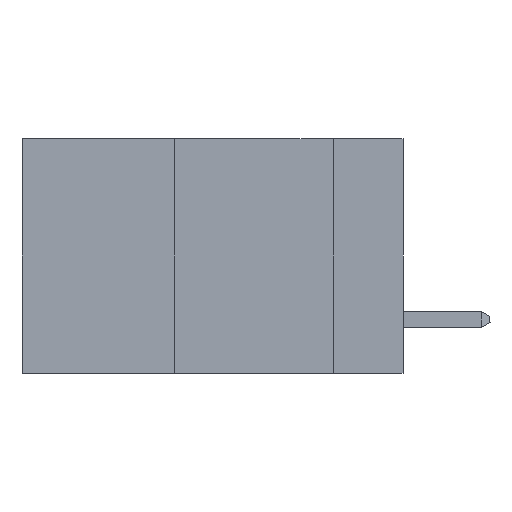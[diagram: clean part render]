
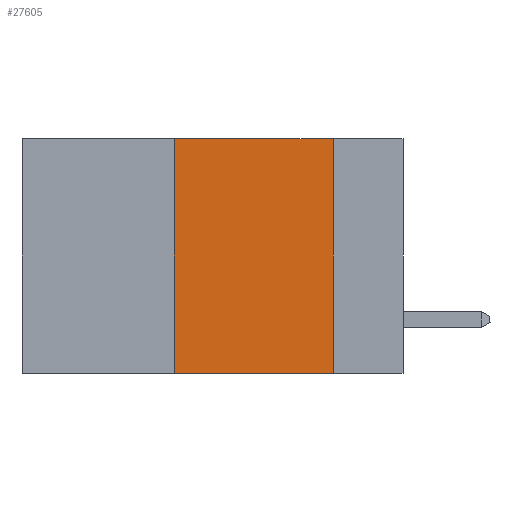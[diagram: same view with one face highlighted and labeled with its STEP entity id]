
A CAD part, left-side view. The second image highlights one B-rep face of the part: STEP entity #27605.
In plain terms, the highlighted planar face has unit normal (-1, 0, 0).
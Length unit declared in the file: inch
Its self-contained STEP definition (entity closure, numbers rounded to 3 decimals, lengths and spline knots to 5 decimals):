
#2439 = EDGE_CURVE ( 'NONE', #4141, #33512, #16038, .T. ) ;
#2485 = EDGE_CURVE ( 'NONE', #33512, #32740, #14207, .T. ) ;
#4136 = FACE_OUTER_BOUND ( 'NONE', #35339, .T. ) ;
#4141 = VERTEX_POINT ( 'NONE', #20916 ) ;
#5521 = DIRECTION ( 'NONE',  ( 1., 0., 0. ) ) ;
#6565 = AXIS2_PLACEMENT_3D ( 'NONE', #14164, #5521, #28145 ) ;
#8400 = EDGE_CURVE ( 'NONE', #13229, #4141, #30937, .T. ) ;
#8492 = VECTOR ( 'NONE', #31058, 39.37008 ) ;
#8522 = ORIENTED_EDGE ( 'NONE', *, *, #31808, .T. ) ;
#10372 = DIRECTION ( 'NONE',  ( 0., -1., 0. ) ) ;
#11355 = DIRECTION ( 'NONE',  ( 0., -1., 0. ) ) ;
#13229 = VERTEX_POINT ( 'NONE', #27263 ) ;
#14164 = CARTESIAN_POINT ( 'NONE',  ( 0., 0.6, 0. ) ) ;
#14207 = LINE ( 'NONE', #33576, #8492 ) ;
#16038 = LINE ( 'NONE', #16825, #27093 ) ;
#16825 = CARTESIAN_POINT ( 'NONE',  ( 0., 0.6, 0. ) ) ;
#16868 = CARTESIAN_POINT ( 'NONE',  ( 0., 0.11, 0. ) ) ;
#17716 = VECTOR ( 'NONE', #10372, 39.37008 ) ;
#20916 = CARTESIAN_POINT ( 'NONE',  ( 0., 0.36, 0. ) ) ;
#22181 = LINE ( 'NONE', #27318, #17716 ) ;
#22459 = PLANE ( 'NONE',  #6565 ) ;
#24068 = CARTESIAN_POINT ( 'NONE',  ( 0., 0.36, 0. ) ) ;
#25558 = ORIENTED_EDGE ( 'NONE', *, *, #2485, .F. ) ;
#27093 = VECTOR ( 'NONE', #11355, 39.37008 ) ;
#27263 = CARTESIAN_POINT ( 'NONE',  ( 0., 0.36, -0.37 ) ) ;
#27318 = CARTESIAN_POINT ( 'NONE',  ( 0., 0.6, -0.37 ) ) ;
#27605 = ADVANCED_FACE ( 'NONE', ( #4136 ), #22459, .F. ) ;
#28145 = DIRECTION ( 'NONE',  ( 0., 0., -1. ) ) ;
#29481 = DIRECTION ( 'NONE',  ( 0., 0., 1. ) ) ;
#29844 = ORIENTED_EDGE ( 'NONE', *, *, #8400, .F. ) ;
#30937 = LINE ( 'NONE', #24068, #33177 ) ;
#31058 = DIRECTION ( 'NONE',  ( 0., 0., -1. ) ) ;
#31808 = EDGE_CURVE ( 'NONE', #13229, #32740, #22181, .T. ) ;
#32740 = VERTEX_POINT ( 'NONE', #35458 ) ;
#33177 = VECTOR ( 'NONE', #29481, 39.37008 ) ;
#33407 = ORIENTED_EDGE ( 'NONE', *, *, #2439, .F. ) ;
#33512 = VERTEX_POINT ( 'NONE', #16868 ) ;
#33576 = CARTESIAN_POINT ( 'NONE',  ( 0., 0.11, 0. ) ) ;
#35339 = EDGE_LOOP ( 'NONE', ( #25558, #33407, #29844, #8522 ) ) ;
#35458 = CARTESIAN_POINT ( 'NONE',  ( 0., 0.11, -0.37 ) ) ;
